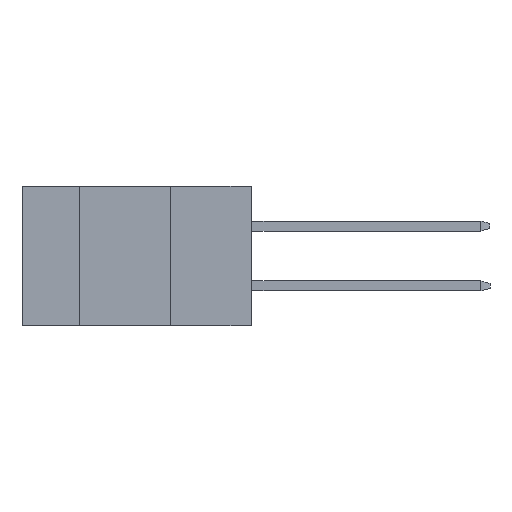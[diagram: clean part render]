
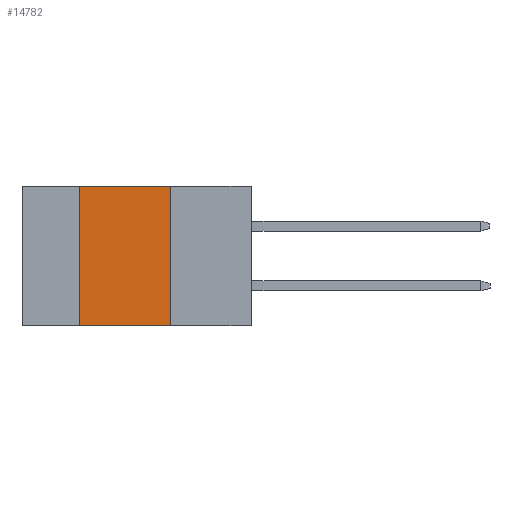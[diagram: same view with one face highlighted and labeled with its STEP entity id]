
A CAD part, left-side view. The second image highlights one B-rep face of the part: STEP entity #14782.
In plain terms, the highlighted planar face has unit normal (-1, 0, 0).
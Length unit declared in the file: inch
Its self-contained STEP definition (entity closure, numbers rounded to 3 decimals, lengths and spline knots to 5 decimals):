
#15 = VERTEX_POINT ( 'NONE', #933 ) ;
#933 = CARTESIAN_POINT ( 'NONE',  ( 0., 0.254, 0. ) ) ;
#1859 = EDGE_CURVE ( 'NONE', #15, #3676, #8681, .T. ) ;
#2304 = LINE ( 'NONE', #13809, #12416 ) ;
#2996 = DIRECTION ( 'NONE',  ( 0., -1., 0. ) ) ;
#3676 = VERTEX_POINT ( 'NONE', #8363 ) ;
#4260 = ORIENTED_EDGE ( 'NONE', *, *, #19732, .F. ) ;
#4985 = CARTESIAN_POINT ( 'NONE',  ( 0., 0.254, -0.437 ) ) ;
#6087 = EDGE_CURVE ( 'NONE', #15011, #3676, #19113, .T. ) ;
#6481 = CARTESIAN_POINT ( 'NONE',  ( 0., 0.54, 0. ) ) ;
#7741 = FACE_OUTER_BOUND ( 'NONE', #18544, .T. ) ;
#8363 = CARTESIAN_POINT ( 'NONE',  ( 0., 0.254, -0.437 ) ) ;
#8681 = LINE ( 'NONE', #4985, #20295 ) ;
#10209 = DIRECTION ( 'NONE',  ( 0., 0., 1. ) ) ;
#10683 = DIRECTION ( 'NONE',  ( 0., 0., -1. ) ) ;
#10707 = ORIENTED_EDGE ( 'NONE', *, *, #15551, .F. ) ;
#11516 = ORIENTED_EDGE ( 'NONE', *, *, #6087, .T. ) ;
#12416 = VECTOR ( 'NONE', #10209, 39.37008 ) ;
#12590 = CARTESIAN_POINT ( 'NONE',  ( 0., 0.72, 0. ) ) ;
#12597 = CARTESIAN_POINT ( 'NONE',  ( 0., 0.72, -0.437 ) ) ;
#13118 = CARTESIAN_POINT ( 'NONE',  ( 0., 0.72, 0. ) ) ;
#13809 = CARTESIAN_POINT ( 'NONE',  ( 0., 0.54, -0.437 ) ) ;
#13967 = PLANE ( 'NONE',  #18850 ) ;
#14388 = VERTEX_POINT ( 'NONE', #6481 ) ;
#14782 = ADVANCED_FACE ( 'NONE', ( #7741 ), #13967, .F. ) ;
#15011 = VERTEX_POINT ( 'NONE', #20239 ) ;
#15024 = DIRECTION ( 'NONE',  ( 0., -1., 0. ) ) ;
#15315 = ORIENTED_EDGE ( 'NONE', *, *, #1859, .F. ) ;
#15551 = EDGE_CURVE ( 'NONE', #15011, #14388, #2304, .T. ) ;
#15630 = VECTOR ( 'NONE', #2996, 39.37008 ) ;
#16572 = LINE ( 'NONE', #13118, #19376 ) ;
#17839 = DIRECTION ( 'NONE',  ( 0., 0., -1. ) ) ;
#18544 = EDGE_LOOP ( 'NONE', ( #15315, #4260, #10707, #11516 ) ) ;
#18687 = DIRECTION ( 'NONE',  ( 1., 0., 0. ) ) ;
#18850 = AXIS2_PLACEMENT_3D ( 'NONE', #12590, #18687, #10683 ) ;
#19113 = LINE ( 'NONE', #12597, #15630 ) ;
#19376 = VECTOR ( 'NONE', #15024, 39.37008 ) ;
#19732 = EDGE_CURVE ( 'NONE', #14388, #15, #16572, .T. ) ;
#20239 = CARTESIAN_POINT ( 'NONE',  ( 0., 0.54, -0.437 ) ) ;
#20295 = VECTOR ( 'NONE', #17839, 39.37008 ) ;
